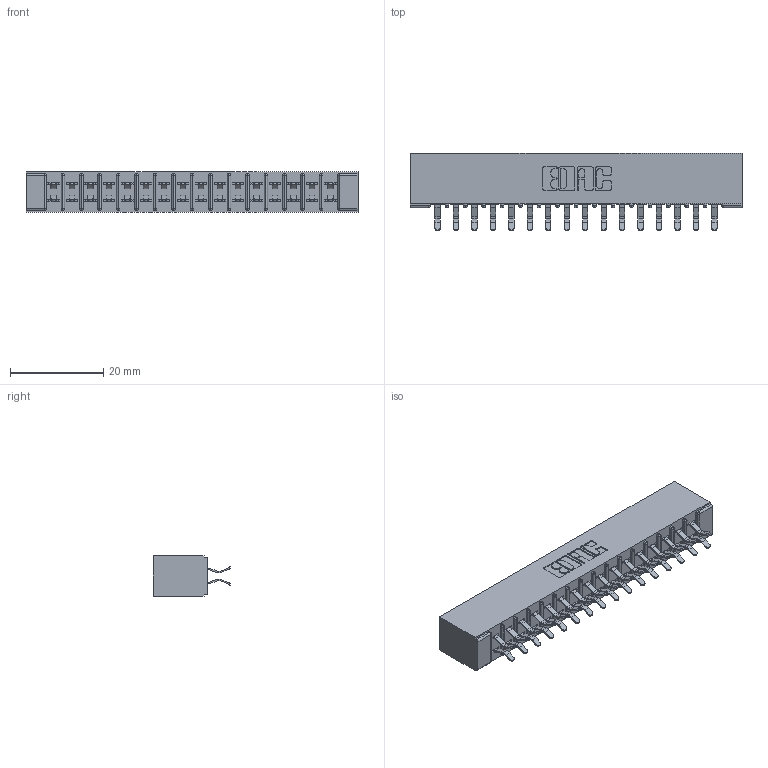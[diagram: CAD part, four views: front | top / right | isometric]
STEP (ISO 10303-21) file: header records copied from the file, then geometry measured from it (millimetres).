
FILE_DESCRIPTION (( 'STEP AP203' ), '1' );
FILE_NAME ('355-032-556-501.STEP', '2019-09-11T08:18:39', ( '' ), ( '' ), 'SwSTEP 2.0', 'SolidWorks 2016', '' );
FILE_SCHEMA (( 'CONFIG_CONTROL_DESIGN' ));
Length unit declared in the file: inch
Products named in the file (3): 355-032-556-501; 305 Part_No Mounting; 305-290-001_556
Assembly tree (33 placements, depth 2):
  355-032-556-501
    305 Part_No Mounting
    305-290-001_556  x32
Bounding box: 71.27 x 16.64 x 8.71 mm (x, y, z)
Volume: 4438.3 mm3; surface area: 9113.5 mm2
Topology: 33 solids, 33 shells, 1900 faces, 5460 edges, 3552 vertices
Faces by surface type: plane 1056, cylinder 780, sphere 64
Entity records: 20433 total; most frequent: CARTESIAN_POINT 3382, ORIENTED_EDGE 3352, DIRECTION 3294, EDGE_CURVE 1676, LINE 1326, VECTOR 1326, VERTEX_POINT 1072, AXIS2_PLACEMENT_3D 984
